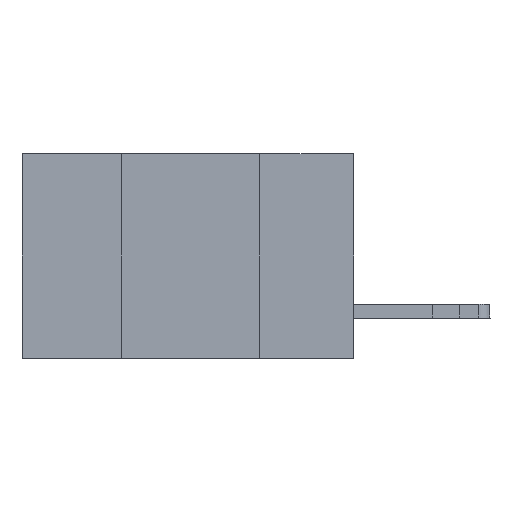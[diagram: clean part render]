
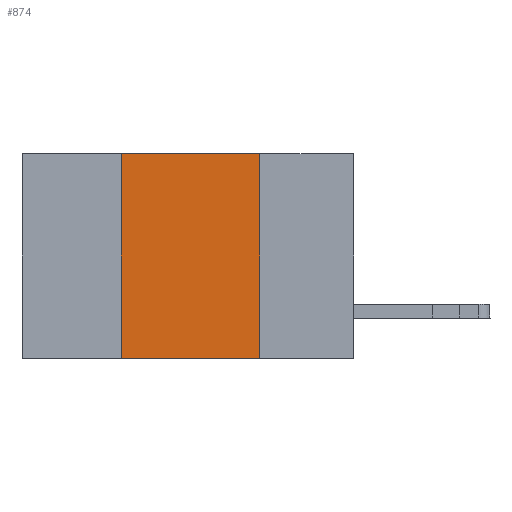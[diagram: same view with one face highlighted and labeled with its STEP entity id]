
A CAD part, left-side view. The second image highlights one B-rep face of the part: STEP entity #874.
In plain terms, the highlighted planar face has unit normal (-1, 0, 0).
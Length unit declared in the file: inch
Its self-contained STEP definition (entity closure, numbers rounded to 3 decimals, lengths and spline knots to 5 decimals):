
#874 = ADVANCED_FACE ( 'NONE', ( #22614 ), #10109, .F. ) ;
#1584 = CARTESIAN_POINT ( 'NONE',  ( 0., 0.42, -0.37 ) ) ;
#2323 = VECTOR ( 'NONE', #23808, 39.37008 ) ;
#2640 = LINE ( 'NONE', #15337, #27872 ) ;
#3395 = AXIS2_PLACEMENT_3D ( 'NONE', #7584, #6850, #11839 ) ;
#6850 = DIRECTION ( 'NONE',  ( 1., 0., 0. ) ) ;
#6928 = DIRECTION ( 'NONE',  ( 0., -1., 0. ) ) ;
#7315 = ORIENTED_EDGE ( 'NONE', *, *, #10977, .F. ) ;
#7584 = CARTESIAN_POINT ( 'NONE',  ( 0., 0.6, 0. ) ) ;
#10109 = PLANE ( 'NONE',  #3395 ) ;
#10977 = EDGE_CURVE ( 'NONE', #24840, #15928, #17749, .T. ) ;
#11138 = CARTESIAN_POINT ( 'NONE',  ( 0., 0.17, -0.37 ) ) ;
#11839 = DIRECTION ( 'NONE',  ( 0., 0., -1. ) ) ;
#14086 = ORIENTED_EDGE ( 'NONE', *, *, #18475, .F. ) ;
#14245 = EDGE_CURVE ( 'NONE', #15928, #20961, #2640, .T. ) ;
#14739 = ORIENTED_EDGE ( 'NONE', *, *, #14245, .F. ) ;
#15292 = ORIENTED_EDGE ( 'NONE', *, *, #31620, .T. ) ;
#15337 = CARTESIAN_POINT ( 'NONE',  ( 0., 0.17, 0. ) ) ;
#15440 = DIRECTION ( 'NONE',  ( 0., 0., -1. ) ) ;
#15928 = VERTEX_POINT ( 'NONE', #21935 ) ;
#17683 = VERTEX_POINT ( 'NONE', #1584 ) ;
#17749 = LINE ( 'NONE', #19686, #23067 ) ;
#18475 = EDGE_CURVE ( 'NONE', #17683, #24840, #20241, .T. ) ;
#19686 = CARTESIAN_POINT ( 'NONE',  ( 0., 0.6, 0. ) ) ;
#20241 = LINE ( 'NONE', #21473, #2323 ) ;
#20961 = VERTEX_POINT ( 'NONE', #11138 ) ;
#21473 = CARTESIAN_POINT ( 'NONE',  ( 0., 0.42, 0. ) ) ;
#21935 = CARTESIAN_POINT ( 'NONE',  ( 0., 0.17, 0. ) ) ;
#22561 = EDGE_LOOP ( 'NONE', ( #14739, #7315, #14086, #15292 ) ) ;
#22614 = FACE_OUTER_BOUND ( 'NONE', #22561, .T. ) ;
#23067 = VECTOR ( 'NONE', #27032, 39.37008 ) ;
#23808 = DIRECTION ( 'NONE',  ( 0., 0., 1. ) ) ;
#24840 = VERTEX_POINT ( 'NONE', #30948 ) ;
#25182 = VECTOR ( 'NONE', #6928, 39.37008 ) ;
#26815 = CARTESIAN_POINT ( 'NONE',  ( 0., 0.6, -0.37 ) ) ;
#27032 = DIRECTION ( 'NONE',  ( 0., -1., 0. ) ) ;
#27481 = LINE ( 'NONE', #26815, #25182 ) ;
#27872 = VECTOR ( 'NONE', #15440, 39.37008 ) ;
#30948 = CARTESIAN_POINT ( 'NONE',  ( 0., 0.42, 0. ) ) ;
#31620 = EDGE_CURVE ( 'NONE', #17683, #20961, #27481, .T. ) ;
